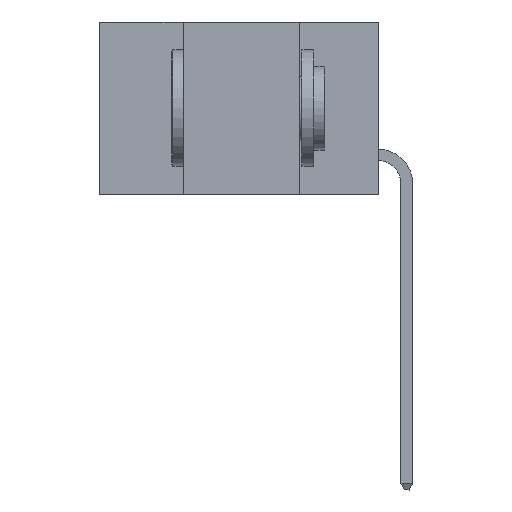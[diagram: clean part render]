
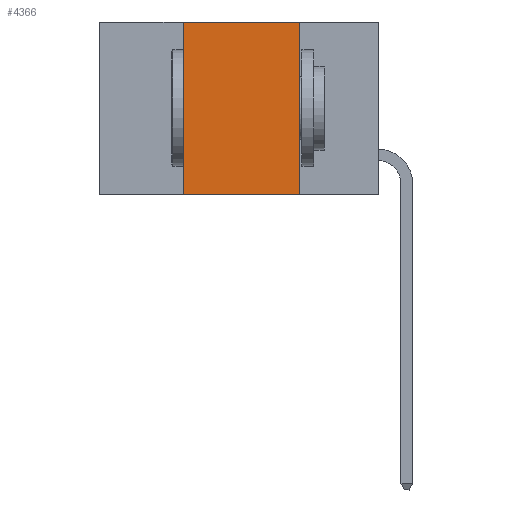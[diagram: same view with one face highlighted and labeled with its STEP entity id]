
A CAD part, left-side view. The second image highlights one B-rep face of the part: STEP entity #4366.
In plain terms, the highlighted planar face has unit normal (-1, 0, 0).
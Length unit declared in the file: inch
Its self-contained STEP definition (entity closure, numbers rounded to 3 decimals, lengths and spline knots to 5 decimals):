
#93 = ORIENTED_EDGE ( 'NONE', *, *, #8369, .F. ) ;
#1290 = DIRECTION ( 'NONE',  ( 0., 0., 1. ) ) ;
#1434 = VECTOR ( 'NONE', #1290, 39.37008 ) ;
#2309 = CARTESIAN_POINT ( 'NONE',  ( 0., 0.42, -0.37 ) ) ;
#2330 = DIRECTION ( 'NONE',  ( 0., -1., 0. ) ) ;
#2524 = EDGE_LOOP ( 'NONE', ( #13235, #93, #5215, #3813 ) ) ;
#2986 = CARTESIAN_POINT ( 'NONE',  ( 0., 0.17, -0.37 ) ) ;
#3320 = LINE ( 'NONE', #2309, #1434 ) ;
#3813 = ORIENTED_EDGE ( 'NONE', *, *, #4356, .T. ) ;
#3875 = EDGE_CURVE ( 'NONE', #13123, #11101, #6951, .T. ) ;
#4216 = VERTEX_POINT ( 'NONE', #7792 ) ;
#4356 = EDGE_CURVE ( 'NONE', #4216, #11101, #6811, .T. ) ;
#4366 = ADVANCED_FACE ( 'NONE', ( #5999 ), #6128, .F. ) ;
#4739 = VECTOR ( 'NONE', #8055, 39.37008 ) ;
#5168 = CARTESIAN_POINT ( 'NONE',  ( 0., 0.17, 0. ) ) ;
#5215 = ORIENTED_EDGE ( 'NONE', *, *, #6863, .F. ) ;
#5798 = VECTOR ( 'NONE', #2330, 39.37008 ) ;
#5801 = CARTESIAN_POINT ( 'NONE',  ( 0., 0.6, -0.37 ) ) ;
#5999 = FACE_OUTER_BOUND ( 'NONE', #2524, .T. ) ;
#6128 = PLANE ( 'NONE',  #13096 ) ;
#6335 = VERTEX_POINT ( 'NONE', #11568 ) ;
#6811 = LINE ( 'NONE', #5801, #4739 ) ;
#6863 = EDGE_CURVE ( 'NONE', #4216, #6335, #3320, .T. ) ;
#6951 = LINE ( 'NONE', #7319, #7617 ) ;
#7082 = CARTESIAN_POINT ( 'NONE',  ( 0., 0.6, 0. ) ) ;
#7319 = CARTESIAN_POINT ( 'NONE',  ( 0., 0.17, -0.37 ) ) ;
#7617 = VECTOR ( 'NONE', #9383, 39.37008 ) ;
#7792 = CARTESIAN_POINT ( 'NONE',  ( 0., 0.42, -0.37 ) ) ;
#8055 = DIRECTION ( 'NONE',  ( 0., -1., 0. ) ) ;
#8369 = EDGE_CURVE ( 'NONE', #6335, #13123, #11710, .T. ) ;
#9097 = DIRECTION ( 'NONE',  ( 0., 0., -1. ) ) ;
#9383 = DIRECTION ( 'NONE',  ( 0., 0., -1. ) ) ;
#9778 = CARTESIAN_POINT ( 'NONE',  ( 0., 0.6, 0. ) ) ;
#11101 = VERTEX_POINT ( 'NONE', #2986 ) ;
#11568 = CARTESIAN_POINT ( 'NONE',  ( 0., 0.42, 0. ) ) ;
#11710 = LINE ( 'NONE', #9778, #5798 ) ;
#13096 = AXIS2_PLACEMENT_3D ( 'NONE', #7082, #13385, #9097 ) ;
#13123 = VERTEX_POINT ( 'NONE', #5168 ) ;
#13235 = ORIENTED_EDGE ( 'NONE', *, *, #3875, .F. ) ;
#13385 = DIRECTION ( 'NONE',  ( 1., 0., 0. ) ) ;
